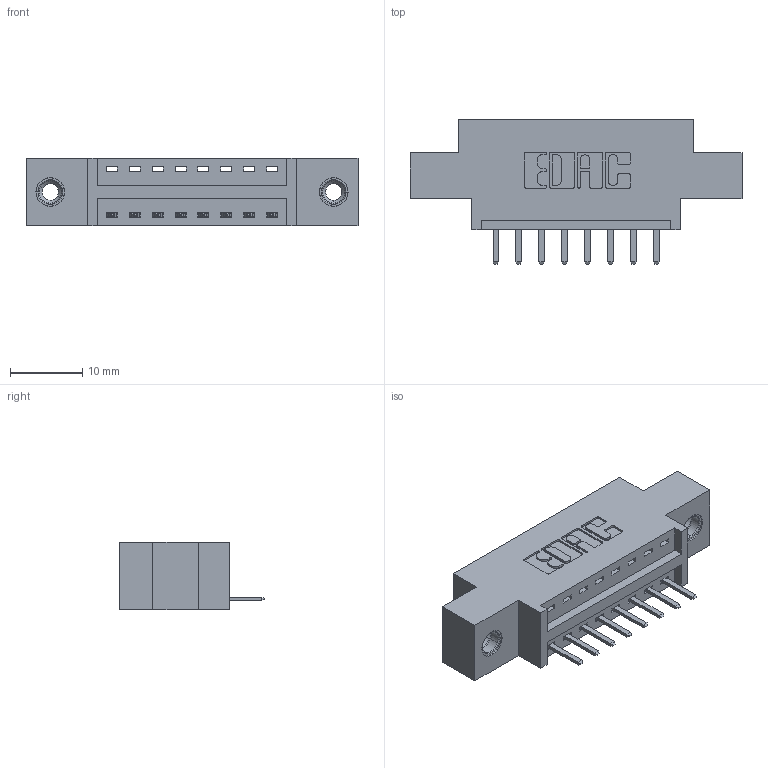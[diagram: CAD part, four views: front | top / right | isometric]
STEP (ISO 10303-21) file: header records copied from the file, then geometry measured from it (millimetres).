
FILE_DESCRIPTION (( 'STEP AP203' ), '1' );
FILE_NAME ('346-008-520-608.STEP', '2018-08-17T04:30:52', ( '' ), ( '' ), 'SwSTEP 2.0', 'SolidWorks 2016', '' );
FILE_SCHEMA (( 'CONFIG_CONTROL_DESIGN' ));
Length unit declared in the file: inch
Products named in the file (4): 345-292-001_345-293-120; 345-250-001_345-250-003-102; 346-008-520-608; 346 Part_0.170 Offset - 0.156 Dia-TI
Assembly tree (11 placements, depth 2):
  346-008-520-608
    346 Part_0.170 Offset - 0.156 Dia-TI
    345-292-001_345-293-120  x8
    345-250-001_345-250-003-102  x2
Bounding box: 45.97 x 20.02 x 9.4 mm (x, y, z)
Volume: 3982.3 mm3; surface area: 4715.8 mm2
Topology: 11 solids, 11 shells, 682 faces, 1949 edges, 1270 vertices
Faces by surface type: plane 448, cylinder 218, cone 12, torus 4
Entity records: 10974 total; most frequent: CARTESIAN_POINT 1887, ORIENTED_EDGE 1810, DIRECTION 1719, EDGE_CURVE 905, LINE 717, VECTOR 717, VERTEX_POINT 596, AXIS2_PLACEMENT_3D 501
